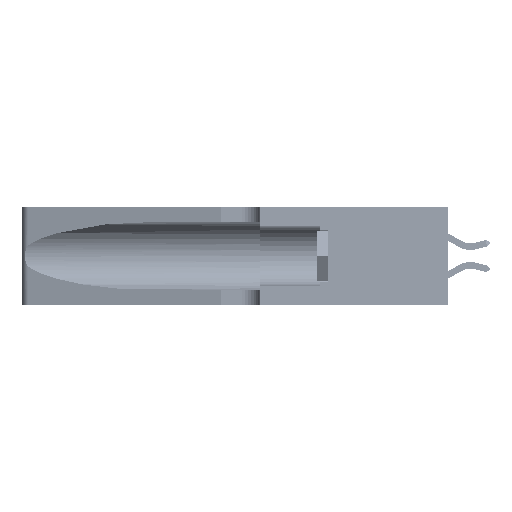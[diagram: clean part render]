
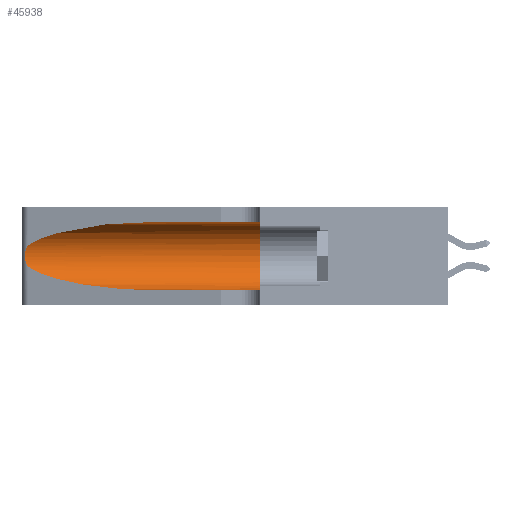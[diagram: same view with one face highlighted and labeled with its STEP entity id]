
A CAD part, left-side view. The second image highlights one B-rep face of the part: STEP entity #45938.
In plain terms, the highlighted cylindrical face has radius 3.308 mm (diameter 6.617 mm), a partial arc.
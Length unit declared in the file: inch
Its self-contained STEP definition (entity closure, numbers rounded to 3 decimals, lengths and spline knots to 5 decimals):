
#311 = CARTESIAN_POINT ( 'NONE',  ( 0.25487, 1.22718, 0.14631 ) ) ;
#447 = VECTOR ( 'NONE', #11161, 39.37008 ) ;
#780 = DIRECTION ( 'NONE',  ( 0., -1., 0. ) ) ;
#1004 = CARTESIAN_POINT ( 'NONE',  ( 0.1305, 0.72297, 0.05475 ) ) ;
#3186 = CARTESIAN_POINT ( 'NONE',  ( 0.25639, 1.23186, 0.15144 ) ) ;
#3714 =( BOUNDED_CURVE ( )  B_SPLINE_CURVE ( 3, ( #47469, #11178, #43593, #1004 ),
 .UNSPECIFIED., .F., .T. ) 
 B_SPLINE_CURVE_WITH_KNOTS ( ( 4, 4 ),
 ( 3.44316, 4.71239 ),
 .UNSPECIFIED. ) 
 CURVE ( )  GEOMETRIC_REPRESENTATION_ITEM ( )  RATIONAL_B_SPLINE_CURVE ( ( 1., 0.87, 0.87, 1. ) ) 
 REPRESENTATION_ITEM ( '' )  );
#5017 = DIRECTION ( 'NONE',  ( 0., 1., 0. ) ) ;
#5710 = VERTEX_POINT ( 'NONE', #34577 ) ;
#6831 = ORIENTED_EDGE ( 'NONE', *, *, #17199, .T. ) ;
#7085 = CARTESIAN_POINT ( 'NONE',  ( 0.2373, 1.15595, 0.28018 ) ) ;
#7432 = CARTESIAN_POINT ( 'NONE',  ( 0.25854, 1.2359, 0.20912 ) ) ;
#8950 = ORIENTED_EDGE ( 'NONE', *, *, #9177, .T. ) ;
#9177 = EDGE_CURVE ( 'NONE', #14573, #29010, #3714, .T. ) ;
#10236 = EDGE_CURVE ( 'NONE', #14914, #5710, #38078, .T. ) ;
#11161 = DIRECTION ( 'NONE',  ( 0., -1., 0. ) ) ;
#11178 = CARTESIAN_POINT ( 'NONE',  ( 0.2373, 1.15595, 0.08982 ) ) ;
#11562 = ORIENTED_EDGE ( 'NONE', *, *, #36297, .F. ) ;
#11635 = CARTESIAN_POINT ( 'NONE',  ( 0.25487, 1.22718, 0.22369 ) ) ;
#11676 = DIRECTION ( 'NONE',  ( 0., -1., 0. ) ) ;
#13358 = ORIENTED_EDGE ( 'NONE', *, *, #18777, .T. ) ;
#14460 = CARTESIAN_POINT ( 'NONE',  ( 0.1305, 0.72297, 0.05475 ) ) ;
#14573 = VERTEX_POINT ( 'NONE', #311 ) ;
#14914 = VERTEX_POINT ( 'NONE', #26824 ) ;
#17199 = EDGE_CURVE ( 'NONE', #25569, #33940, #49108, .T. ) ;
#17713 = CARTESIAN_POINT ( 'NONE',  ( 0.1305, 0.35, 0.185 ) ) ;
#18647 = FACE_OUTER_BOUND ( 'NONE', #42847, .T. ) ;
#18777 = EDGE_CURVE ( 'NONE', #29010, #5710, #26414, .T. ) ;
#18938 = CARTESIAN_POINT ( 'NONE',  ( 0.26075, 1.23896, 0.19203 ) ) ;
#19338 = CARTESIAN_POINT ( 'NONE',  ( 0.1305, 1.61858, 0.05475 ) ) ;
#23381 = CARTESIAN_POINT ( 'NONE',  ( 0.26018, 1.23835, 0.19895 ) ) ;
#23387 = CARTESIAN_POINT ( 'NONE',  ( 0.18966, 0.96281, 0.31525 ) ) ;
#23552 = CARTESIAN_POINT ( 'NONE',  ( 0.26017, 1.23833, 0.17102 ) ) ;
#24151 = B_SPLINE_CURVE_WITH_KNOTS ( 'NONE', 3,
 ( #43184, #27446, #31512, #51136, #7432, #23381, #18938, #51667, #23552, #27265, #35755, #3186, #47236, #51494 ),
 .UNSPECIFIED., .F., .F.,
 ( 4, 2, 2, 2, 2, 2, 4 ),
 ( 0., 0.00027, 0.00053, 0.00107, 0.0016, 0.00187, 0.00214 ),
 .UNSPECIFIED. ) ;
#25569 = VERTEX_POINT ( 'NONE', #47982 ) ;
#26414 = LINE ( 'NONE', #19338, #447 ) ;
#26499 = EDGE_CURVE ( 'NONE', #33940, #14573, #24151, .T. ) ;
#26824 = CARTESIAN_POINT ( 'NONE',  ( 0.1305, 0.35, 0.31525 ) ) ;
#27265 = CARTESIAN_POINT ( 'NONE',  ( 0.25856, 1.23593, 0.16098 ) ) ;
#27271 = CARTESIAN_POINT ( 'NONE',  ( 0.1305, 0.72297, 0.31525 ) ) ;
#27446 = CARTESIAN_POINT ( 'NONE',  ( 0.25555, 1.22994, 0.2215 ) ) ;
#28382 = CARTESIAN_POINT ( 'NONE',  ( 0.1305, 1.61858, 0.31525 ) ) ;
#29010 = VERTEX_POINT ( 'NONE', #14460 ) ;
#29441 = VECTOR ( 'NONE', #780, 39.37008 ) ;
#31512 = CARTESIAN_POINT ( 'NONE',  ( 0.25639, 1.23184, 0.21858 ) ) ;
#33940 = VERTEX_POINT ( 'NONE', #11635 ) ;
#34577 = CARTESIAN_POINT ( 'NONE',  ( 0.1305, 0.35, 0.05475 ) ) ;
#35407 = CARTESIAN_POINT ( 'NONE',  ( 0.25487, 1.22718, 0.22369 ) ) ;
#35755 = CARTESIAN_POINT ( 'NONE',  ( 0.25789, 1.23486, 0.15765 ) ) ;
#35796 = CARTESIAN_POINT ( 'NONE',  ( 0.1305, 1.61858, 0.185 ) ) ;
#36297 = EDGE_CURVE ( 'NONE', #25569, #14914, #51593, .T. ) ;
#37229 = DIRECTION ( 'NONE',  ( 0., 0., 1. ) ) ;
#37645 = CYLINDRICAL_SURFACE ( 'NONE', #39170, 0.13025 ) ;
#38078 = CIRCLE ( 'NONE', #38144, 0.13025 ) ;
#38144 = AXIS2_PLACEMENT_3D ( 'NONE', #17713, #5017, #37229 ) ;
#39170 = AXIS2_PLACEMENT_3D ( 'NONE', #35796, #11676, #43918 ) ;
#42847 = EDGE_LOOP ( 'NONE', ( #6831, #47840, #8950, #13358, #43301, #11562 ) ) ;
#43184 = CARTESIAN_POINT ( 'NONE',  ( 0.25487, 1.22718, 0.22369 ) ) ;
#43301 = ORIENTED_EDGE ( 'NONE', *, *, #10236, .F. ) ;
#43593 = CARTESIAN_POINT ( 'NONE',  ( 0.18966, 0.96281, 0.05475 ) ) ;
#43918 = DIRECTION ( 'NONE',  ( 0., 0., -1. ) ) ;
#45938 = ADVANCED_FACE ( 'NONE', ( #18647 ), #37645, .F. ) ;
#47236 = CARTESIAN_POINT ( 'NONE',  ( 0.25555, 1.22993, 0.14849 ) ) ;
#47469 = CARTESIAN_POINT ( 'NONE',  ( 0.25487, 1.22718, 0.14631 ) ) ;
#47840 = ORIENTED_EDGE ( 'NONE', *, *, #26499, .T. ) ;
#47982 = CARTESIAN_POINT ( 'NONE',  ( 0.1305, 0.72297, 0.31525 ) ) ;
#49108 =( BOUNDED_CURVE ( )  B_SPLINE_CURVE ( 3, ( #27271, #23387, #7085, #35407 ),
 .UNSPECIFIED., .F., .F. ) 
 B_SPLINE_CURVE_WITH_KNOTS ( ( 4, 4 ),
 ( 1.5708, 2.84003 ),
 .UNSPECIFIED. ) 
 CURVE ( )  GEOMETRIC_REPRESENTATION_ITEM ( )  RATIONAL_B_SPLINE_CURVE ( ( 1., 0.87, 0.87, 1. ) ) 
 REPRESENTATION_ITEM ( '' )  );
#51136 = CARTESIAN_POINT ( 'NONE',  ( 0.25787, 1.23484, 0.2124 ) ) ;
#51494 = CARTESIAN_POINT ( 'NONE',  ( 0.25487, 1.22718, 0.14631 ) ) ;
#51593 = LINE ( 'NONE', #28382, #29441 ) ;
#51667 = CARTESIAN_POINT ( 'NONE',  ( 0.26075, 1.23896, 0.178 ) ) ;
